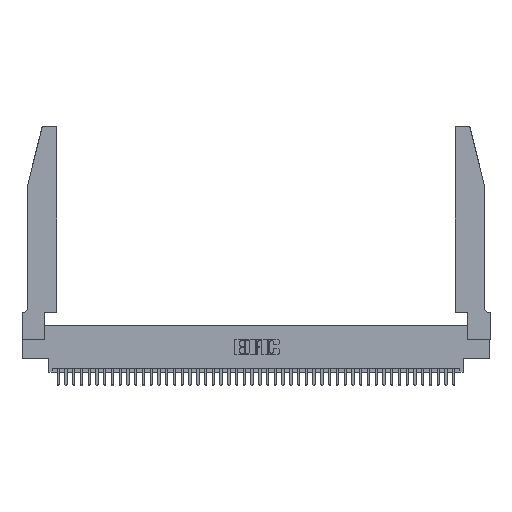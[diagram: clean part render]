
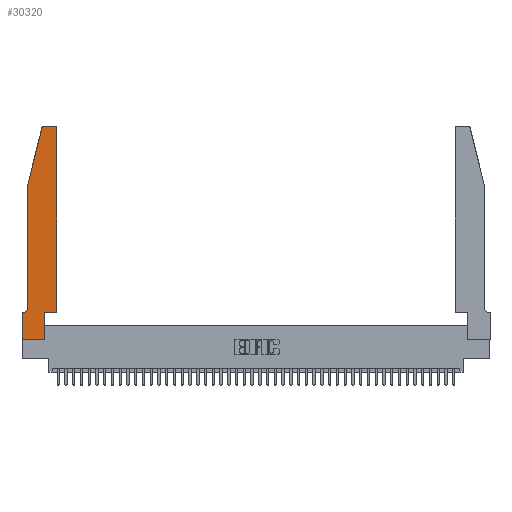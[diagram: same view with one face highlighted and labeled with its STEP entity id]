
A CAD part, top view. The second image highlights one B-rep face of the part: STEP entity #30320.
In plain terms, the highlighted planar face has unit normal (0, 0, 1).
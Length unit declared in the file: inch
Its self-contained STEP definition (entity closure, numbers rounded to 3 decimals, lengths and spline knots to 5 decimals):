
#681 = VECTOR ( 'NONE', #26253, 39.37008 ) ;
#811 = ORIENTED_EDGE ( 'NONE', *, *, #18369, .T. ) ;
#1244 = CARTESIAN_POINT ( 'NONE',  ( 0.0755, 2., 0.37 ) ) ;
#1264 = VECTOR ( 'NONE', #35611, 39.37008 ) ;
#2219 = CARTESIAN_POINT ( 'NONE',  ( 0.4505, 0.35, 0.37 ) ) ;
#2453 = VECTOR ( 'NONE', #41000, 39.37008 ) ;
#2536 = AXIS2_PLACEMENT_3D ( 'NONE', #34281, #13764, #37733 ) ;
#2697 = DIRECTION ( 'NONE',  ( 0., 0., 1. ) ) ;
#3647 = CARTESIAN_POINT ( 'NONE',  ( 0.0055, 0.42, 0.37 ) ) ;
#3732 = ORIENTED_EDGE ( 'NONE', *, *, #6015, .T. ) ;
#3840 = EDGE_CURVE ( 'NONE', #17764, #42388, #7863, .T. ) ;
#3968 = EDGE_CURVE ( 'NONE', #42410, #41192, #40072, .T. ) ;
#4240 = LINE ( 'NONE', #30812, #39673 ) ;
#4906 = CARTESIAN_POINT ( 'NONE',  ( 0.2865, 0., 0.37 ) ) ;
#4973 = ORIENTED_EDGE ( 'NONE', *, *, #3840, .T. ) ;
#6015 = EDGE_CURVE ( 'NONE', #31247, #7873, #39952, .T. ) ;
#6734 = VECTOR ( 'NONE', #25770, 39.37008 ) ;
#7099 = DIRECTION ( 'NONE',  ( -1., 0., 0. ) ) ;
#7143 = ORIENTED_EDGE ( 'NONE', *, *, #31767, .T. ) ;
#7667 = CARTESIAN_POINT ( 'NONE',  ( 0.4505, 0.35, 0.37 ) ) ;
#7863 = CIRCLE ( 'NONE', #15705, 0.03 ) ;
#7873 = VERTEX_POINT ( 'NONE', #31582 ) ;
#9124 = CARTESIAN_POINT ( 'NONE',  ( 0.284, 2.75, 0.37 ) ) ;
#10312 = CARTESIAN_POINT ( 'NONE',  ( 0.4205, 2.75, 0.37 ) ) ;
#10794 = VERTEX_POINT ( 'NONE', #10312 ) ;
#10984 = VERTEX_POINT ( 'NONE', #28583 ) ;
#11371 = CARTESIAN_POINT ( 'NONE',  ( 0.2865, 0.35, 0.37 ) ) ;
#11506 = LINE ( 'NONE', #32185, #1264 ) ;
#11778 = ORIENTED_EDGE ( 'NONE', *, *, #37294, .T. ) ;
#12161 = LINE ( 'NONE', #11371, #29320 ) ;
#13549 = CARTESIAN_POINT ( 'NONE',  ( 0.0755, 2., 0.37 ) ) ;
#13764 = DIRECTION ( 'NONE',  ( 0., 0., 1. ) ) ;
#14150 = VERTEX_POINT ( 'NONE', #29801 ) ;
#14593 = EDGE_CURVE ( 'NONE', #42388, #42410, #38874, .T. ) ;
#14598 = EDGE_CURVE ( 'NONE', #7873, #14150, #11506, .T. ) ;
#14683 = AXIS2_PLACEMENT_3D ( 'NONE', #30668, #44344, #37590 ) ;
#15476 = CARTESIAN_POINT ( 'NONE',  ( 0.2605, 2.75, 0.37 ) ) ;
#15543 = FACE_OUTER_BOUND ( 'NONE', #19910, .T. ) ;
#15705 = AXIS2_PLACEMENT_3D ( 'NONE', #23254, #2697, #26714 ) ;
#17764 = VERTEX_POINT ( 'NONE', #9124 ) ;
#18057 = ORIENTED_EDGE ( 'NONE', *, *, #29592, .T. ) ;
#18369 = EDGE_CURVE ( 'NONE', #39264, #27345, #4240, .T. ) ;
#18389 = DIRECTION ( 'NONE',  ( -0.239, -0.971, 0. ) ) ;
#18755 = CARTESIAN_POINT ( 'NONE',  ( 0.0055, 0.35, 0.37 ) ) ;
#19554 = VECTOR ( 'NONE', #18389, 39.37008 ) ;
#19904 = VERTEX_POINT ( 'NONE', #4906 ) ;
#19910 = EDGE_LOOP ( 'NONE', ( #25626, #4973, #28620, #34307, #31091, #3732, #28460, #11778, #7143, #32015, #811, #18057 ) ) ;
#20472 = DIRECTION ( 'NONE',  ( 0., 1., 0. ) ) ;
#21077 = DIRECTION ( 'NONE',  ( 1., 0., 0. ) ) ;
#21661 = VECTOR ( 'NONE', #21077, 39.37008 ) ;
#21980 = EDGE_CURVE ( 'NONE', #10794, #17764, #42187, .T. ) ;
#23254 = CARTESIAN_POINT ( 'NONE',  ( 0.284, 2.72, 0.37 ) ) ;
#24154 = CIRCLE ( 'NONE', #2536, 0.03 ) ;
#24312 = CARTESIAN_POINT ( 'NONE',  ( 0.0755, 0.35, 0.37 ) ) ;
#25146 = DIRECTION ( 'NONE',  ( 0., 1., 0. ) ) ;
#25626 = ORIENTED_EDGE ( 'NONE', *, *, #21980, .T. ) ;
#25770 = DIRECTION ( 'NONE',  ( -1., 0., 0. ) ) ;
#26253 = DIRECTION ( 'NONE',  ( 1., 0., 0. ) ) ;
#26714 = DIRECTION ( 'NONE',  ( 1., 0., 0. ) ) ;
#27015 = LINE ( 'NONE', #2219, #681 ) ;
#27345 = VERTEX_POINT ( 'NONE', #38978 ) ;
#27668 = DIRECTION ( 'NONE',  ( 0., 0., -1. ) ) ;
#28460 = ORIENTED_EDGE ( 'NONE', *, *, #14598, .T. ) ;
#28583 = CARTESIAN_POINT ( 'NONE',  ( 0.2865, 0.35, 0.37 ) ) ;
#28620 = ORIENTED_EDGE ( 'NONE', *, *, #14593, .T. ) ;
#29320 = VECTOR ( 'NONE', #25146, 39.37008 ) ;
#29592 = EDGE_CURVE ( 'NONE', #27345, #10794, #24154, .T. ) ;
#29801 = CARTESIAN_POINT ( 'NONE',  ( 0., 0., 0.37 ) ) ;
#30320 = ADVANCED_FACE ( 'NONE', ( #15543 ), #34132, .T. ) ;
#30668 = CARTESIAN_POINT ( 'NONE',  ( 0., 0.35, 0.37 ) ) ;
#30805 = VECTOR ( 'NONE', #31201, 39.37008 ) ;
#30812 = CARTESIAN_POINT ( 'NONE',  ( 0.4505, 0.35, 0.37 ) ) ;
#31091 = ORIENTED_EDGE ( 'NONE', *, *, #35839, .T. ) ;
#31201 = DIRECTION ( 'NONE',  ( -1., 0., 0. ) ) ;
#31247 = VERTEX_POINT ( 'NONE', #18755 ) ;
#31582 = CARTESIAN_POINT ( 'NONE',  ( 0., 0.35, 0.37 ) ) ;
#31767 = EDGE_CURVE ( 'NONE', #19904, #10984, #12161, .T. ) ;
#31828 = CARTESIAN_POINT ( 'NONE',  ( 0.25487, 2.72718, 0.37 ) ) ;
#32015 = ORIENTED_EDGE ( 'NONE', *, *, #41469, .T. ) ;
#32185 = CARTESIAN_POINT ( 'NONE',  ( 0., 0., 0.37 ) ) ;
#34132 = PLANE ( 'NONE',  #14683 ) ;
#34281 = CARTESIAN_POINT ( 'NONE',  ( 0.4205, 2.72, 0.37 ) ) ;
#34307 = ORIENTED_EDGE ( 'NONE', *, *, #3968, .T. ) ;
#35611 = DIRECTION ( 'NONE',  ( 0., -1., 0. ) ) ;
#35839 = EDGE_CURVE ( 'NONE', #41192, #31247, #40077, .T. ) ;
#37294 = EDGE_CURVE ( 'NONE', #14150, #19904, #39947, .T. ) ;
#37590 = DIRECTION ( 'NONE',  ( 1., 0., 0. ) ) ;
#37733 = DIRECTION ( 'NONE',  ( 1., 0., 0. ) ) ;
#38874 = LINE ( 'NONE', #1244, #19554 ) ;
#38978 = CARTESIAN_POINT ( 'NONE',  ( 0.4505, 2.72, 0.37 ) ) ;
#39264 = VERTEX_POINT ( 'NONE', #7667 ) ;
#39673 = VECTOR ( 'NONE', #20472, 39.37008 ) ;
#39947 = LINE ( 'NONE', #41678, #21661 ) ;
#39952 = LINE ( 'NONE', #24312, #30805 ) ;
#40072 = LINE ( 'NONE', #13549, #2453 ) ;
#40077 = CIRCLE ( 'NONE', #43247, 0.07 ) ;
#41000 = DIRECTION ( 'NONE',  ( 0., -1., 0. ) ) ;
#41192 = VERTEX_POINT ( 'NONE', #41898 ) ;
#41469 = EDGE_CURVE ( 'NONE', #10984, #39264, #27015, .T. ) ;
#41678 = CARTESIAN_POINT ( 'NONE',  ( 0., 0., 0.37 ) ) ;
#41898 = CARTESIAN_POINT ( 'NONE',  ( 0.0755, 0.42, 0.37 ) ) ;
#42062 = CARTESIAN_POINT ( 'NONE',  ( 0.0755, 2., 0.37 ) ) ;
#42187 = LINE ( 'NONE', #15476, #6734 ) ;
#42388 = VERTEX_POINT ( 'NONE', #31828 ) ;
#42410 = VERTEX_POINT ( 'NONE', #42062 ) ;
#43247 = AXIS2_PLACEMENT_3D ( 'NONE', #3647, #27668, #7099 ) ;
#44344 = DIRECTION ( 'NONE',  ( 0., 0., 1. ) ) ;
